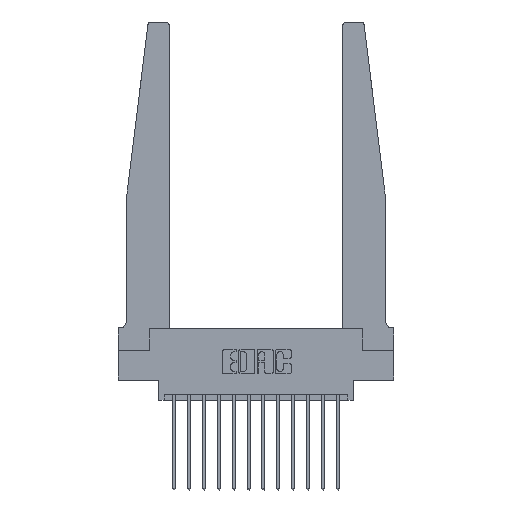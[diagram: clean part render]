
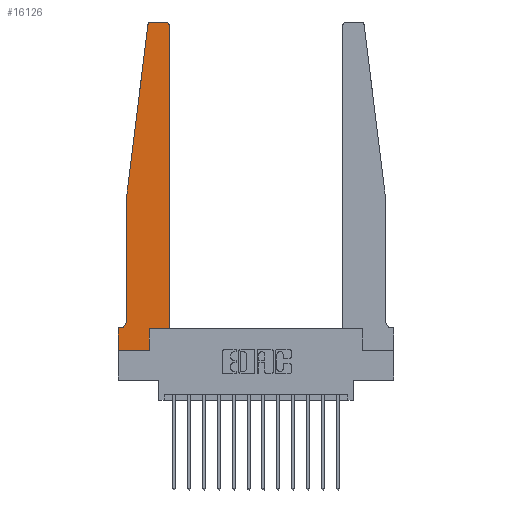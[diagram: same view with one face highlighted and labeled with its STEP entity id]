
A CAD part, top view. The second image highlights one B-rep face of the part: STEP entity #16126.
In plain terms, the highlighted planar face has unit normal (0, 0, 1).
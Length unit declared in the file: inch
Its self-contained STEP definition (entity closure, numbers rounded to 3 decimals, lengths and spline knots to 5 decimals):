
#180 = LINE ( 'NONE', #13575, #7099 ) ;
#282 = CARTESIAN_POINT ( 'NONE',  ( 0.24675, 2.72367, 0.37 ) ) ;
#517 = CARTESIAN_POINT ( 'NONE',  ( 0., 0., 0.37 ) ) ;
#795 = ORIENTED_EDGE ( 'NONE', *, *, #10935, .T. ) ;
#870 = DIRECTION ( 'NONE',  ( 0., 1., 0. ) ) ;
#1028 = EDGE_CURVE ( 'NONE', #3606, #2430, #15058, .T. ) ;
#1052 = CARTESIAN_POINT ( 'NONE',  ( 0.2605, 0.18, 0.37 ) ) ;
#1146 = ORIENTED_EDGE ( 'NONE', *, *, #15884, .T. ) ;
#1447 = CIRCLE ( 'NONE', #9543, 0.03 ) ;
#1918 = EDGE_CURVE ( 'NONE', #7833, #9878, #13191, .T. ) ;
#1926 = LINE ( 'NONE', #13391, #7987 ) ;
#1989 = VERTEX_POINT ( 'NONE', #15163 ) ;
#2138 = DIRECTION ( 'NONE',  ( 0., 0., 1. ) ) ;
#2289 = LINE ( 'NONE', #16407, #12195 ) ;
#2430 = VERTEX_POINT ( 'NONE', #517 ) ;
#2575 = CARTESIAN_POINT ( 'NONE',  ( 0., 0., 0.37 ) ) ;
#2782 = CARTESIAN_POINT ( 'NONE',  ( 0.065, 1.25, 0.37 ) ) ;
#2801 = ORIENTED_EDGE ( 'NONE', *, *, #15774, .T. ) ;
#3025 = ORIENTED_EDGE ( 'NONE', *, *, #13361, .T. ) ;
#3181 = CARTESIAN_POINT ( 'NONE',  ( 0.27653, 2.72, 0.37 ) ) ;
#3370 = DIRECTION ( 'NONE',  ( 0., 0., -1. ) ) ;
#3407 = CARTESIAN_POINT ( 'NONE',  ( 0.25, 2.75, 0.37 ) ) ;
#3447 = VECTOR ( 'NONE', #16623, 39.37008 ) ;
#3458 = VERTEX_POINT ( 'NONE', #10591 ) ;
#3606 = VERTEX_POINT ( 'NONE', #12163 ) ;
#3616 = VERTEX_POINT ( 'NONE', #4481 ) ;
#3632 = EDGE_CURVE ( 'NONE', #10264, #3606, #180, .T. ) ;
#3661 = EDGE_LOOP ( 'NONE', ( #1146, #2801, #6439, #795, #6294, #13067, #4536, #14632, #15336, #3025, #16317, #6005 ) ) ;
#3696 = LINE ( 'NONE', #13735, #6741 ) ;
#3862 = EDGE_CURVE ( 'NONE', #3458, #1989, #13750, .T. ) ;
#3985 = CARTESIAN_POINT ( 'NONE',  ( 0.425, 0.18, 0.37 ) ) ;
#3998 = DIRECTION ( 'NONE',  ( 0., -1., 0. ) ) ;
#4093 = DIRECTION ( 'NONE',  ( -0.122, -0.992, 0. ) ) ;
#4298 = CARTESIAN_POINT ( 'NONE',  ( 0., 0.1875, 0.37 ) ) ;
#4481 = CARTESIAN_POINT ( 'NONE',  ( 0.27653, 2.75, 0.37 ) ) ;
#4482 = DIRECTION ( 'NONE',  ( 1., 0., 0. ) ) ;
#4536 = ORIENTED_EDGE ( 'NONE', *, *, #1028, .T. ) ;
#4539 = DIRECTION ( 'NONE',  ( -1., 0., 0. ) ) ;
#5612 = DIRECTION ( 'NONE',  ( 1., 0., 0. ) ) ;
#6005 = ORIENTED_EDGE ( 'NONE', *, *, #1918, .T. ) ;
#6294 = ORIENTED_EDGE ( 'NONE', *, *, #10159, .T. ) ;
#6439 = ORIENTED_EDGE ( 'NONE', *, *, #10474, .T. ) ;
#6741 = VECTOR ( 'NONE', #12430, 39.37008 ) ;
#7099 = VECTOR ( 'NONE', #4539, 39.37008 ) ;
#7382 = AXIS2_PLACEMENT_3D ( 'NONE', #9912, #2138, #11205 ) ;
#7833 = VERTEX_POINT ( 'NONE', #11677 ) ;
#7840 = VECTOR ( 'NONE', #12723, 39.37008 ) ;
#7987 = VECTOR ( 'NONE', #16008, 39.37008 ) ;
#8164 = VECTOR ( 'NONE', #3998, 39.37008 ) ;
#8221 = VERTEX_POINT ( 'NONE', #11220 ) ;
#8733 = CARTESIAN_POINT ( 'NONE',  ( 0.015, 0.1875, 0.37 ) ) ;
#8858 = EDGE_CURVE ( 'NONE', #12258, #7833, #2289, .T. ) ;
#9150 = CARTESIAN_POINT ( 'NONE',  ( 0.065, 1.25, 0.37 ) ) ;
#9209 = AXIS2_PLACEMENT_3D ( 'NONE', #4298, #13337, #5612 ) ;
#9353 = VECTOR ( 'NONE', #9918, 39.37008 ) ;
#9543 = AXIS2_PLACEMENT_3D ( 'NONE', #3181, #12219, #4482 ) ;
#9820 = CARTESIAN_POINT ( 'NONE',  ( 0.395, 2.75, 0.37 ) ) ;
#9878 = VERTEX_POINT ( 'NONE', #9820 ) ;
#9912 = CARTESIAN_POINT ( 'NONE',  ( 0.395, 2.72, 0.37 ) ) ;
#9918 = DIRECTION ( 'NONE',  ( -1., 0., 0. ) ) ;
#10158 = LINE ( 'NONE', #3407, #9353 ) ;
#10159 = EDGE_CURVE ( 'NONE', #8221, #10264, #15807, .T. ) ;
#10264 = VERTEX_POINT ( 'NONE', #8733 ) ;
#10474 = EDGE_CURVE ( 'NONE', #11853, #13813, #13942, .T. ) ;
#10591 = CARTESIAN_POINT ( 'NONE',  ( 0.2605, 0., 0.37 ) ) ;
#10935 = EDGE_CURVE ( 'NONE', #13813, #8221, #11700, .T. ) ;
#11124 = CARTESIAN_POINT ( 'NONE',  ( 0.015, 0.2375, 0.37 ) ) ;
#11205 = DIRECTION ( 'NONE',  ( 1., 0., 0. ) ) ;
#11220 = CARTESIAN_POINT ( 'NONE',  ( 0.065, 0.2375, 0.37 ) ) ;
#11423 = CARTESIAN_POINT ( 'NONE',  ( 0.065, 1.25, 0.37 ) ) ;
#11677 = CARTESIAN_POINT ( 'NONE',  ( 0.425, 2.72, 0.37 ) ) ;
#11700 = LINE ( 'NONE', #11423, #7840 ) ;
#11853 = VERTEX_POINT ( 'NONE', #282 ) ;
#12041 = PLANE ( 'NONE',  #9209 ) ;
#12163 = CARTESIAN_POINT ( 'NONE',  ( 0., 0.1875, 0.37 ) ) ;
#12195 = VECTOR ( 'NONE', #870, 39.37008 ) ;
#12219 = DIRECTION ( 'NONE',  ( 0., 0., 1. ) ) ;
#12258 = VERTEX_POINT ( 'NONE', #3985 ) ;
#12391 = AXIS2_PLACEMENT_3D ( 'NONE', #11124, #3370, #12405 ) ;
#12405 = DIRECTION ( 'NONE',  ( -1., 0., 0. ) ) ;
#12430 = DIRECTION ( 'NONE',  ( 1., 0., 0. ) ) ;
#12723 = DIRECTION ( 'NONE',  ( 0., -1., 0. ) ) ;
#13067 = ORIENTED_EDGE ( 'NONE', *, *, #3632, .T. ) ;
#13191 = CIRCLE ( 'NONE', #7382, 0.03 ) ;
#13337 = DIRECTION ( 'NONE',  ( 0., 0., 1. ) ) ;
#13361 = EDGE_CURVE ( 'NONE', #1989, #12258, #1926, .T. ) ;
#13391 = CARTESIAN_POINT ( 'NONE',  ( 0.425, 0.18, 0.37 ) ) ;
#13531 = VECTOR ( 'NONE', #4093, 39.37008 ) ;
#13575 = CARTESIAN_POINT ( 'NONE',  ( 0.065, 0.1875, 0.37 ) ) ;
#13735 = CARTESIAN_POINT ( 'NONE',  ( 0., 0., 0.37 ) ) ;
#13750 = LINE ( 'NONE', #1052, #3447 ) ;
#13813 = VERTEX_POINT ( 'NONE', #9150 ) ;
#13942 = LINE ( 'NONE', #2782, #13531 ) ;
#14632 = ORIENTED_EDGE ( 'NONE', *, *, #15353, .T. ) ;
#15058 = LINE ( 'NONE', #2575, #8164 ) ;
#15163 = CARTESIAN_POINT ( 'NONE',  ( 0.2605, 0.18, 0.37 ) ) ;
#15336 = ORIENTED_EDGE ( 'NONE', *, *, #3862, .T. ) ;
#15353 = EDGE_CURVE ( 'NONE', #2430, #3458, #3696, .T. ) ;
#15774 = EDGE_CURVE ( 'NONE', #3616, #11853, #1447, .T. ) ;
#15807 = CIRCLE ( 'NONE', #12391, 0.05 ) ;
#15884 = EDGE_CURVE ( 'NONE', #9878, #3616, #10158, .T. ) ;
#16008 = DIRECTION ( 'NONE',  ( 1., 0., 0. ) ) ;
#16126 = ADVANCED_FACE ( 'NONE', ( #16421 ), #12041, .T. ) ;
#16317 = ORIENTED_EDGE ( 'NONE', *, *, #8858, .T. ) ;
#16407 = CARTESIAN_POINT ( 'NONE',  ( 0.425, 0.18, 0.37 ) ) ;
#16421 = FACE_OUTER_BOUND ( 'NONE', #3661, .T. ) ;
#16623 = DIRECTION ( 'NONE',  ( 0., 1., 0. ) ) ;
